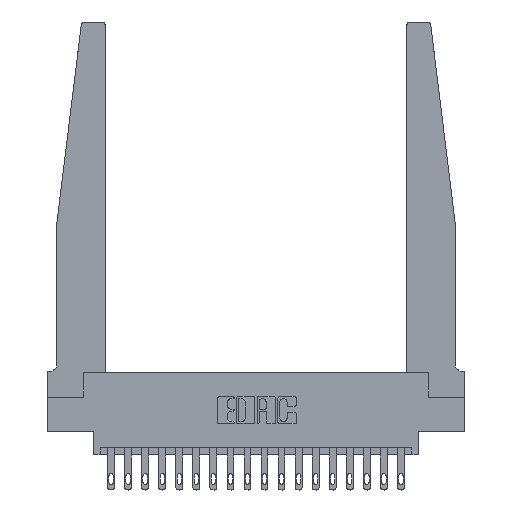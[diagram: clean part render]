
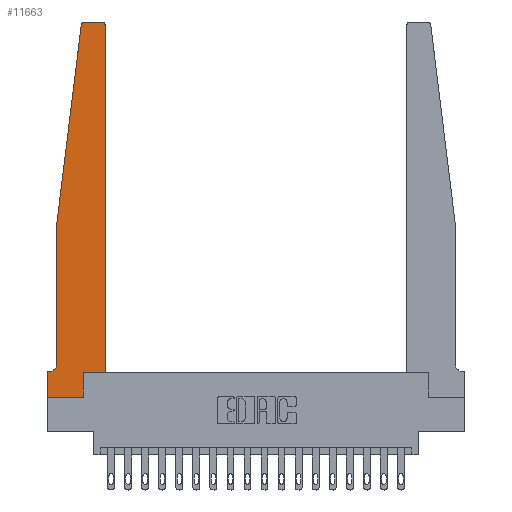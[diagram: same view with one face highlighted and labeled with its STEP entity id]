
A CAD part, top view. The second image highlights one B-rep face of the part: STEP entity #11663.
In plain terms, the highlighted planar face has unit normal (0, 0, 1).
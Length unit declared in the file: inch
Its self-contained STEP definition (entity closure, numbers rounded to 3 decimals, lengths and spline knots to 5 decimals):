
#493 = CARTESIAN_POINT ( 'NONE',  ( 0.425, 0.18, 0.37 ) ) ;
#527 = ORIENTED_EDGE ( 'NONE', *, *, #17623, .T. ) ;
#646 = LINE ( 'NONE', #11451, #14542 ) ;
#763 = LINE ( 'NONE', #2199, #16998 ) ;
#764 = LINE ( 'NONE', #10218, #9113 ) ;
#1046 = DIRECTION ( 'NONE',  ( 0., 0., 1. ) ) ;
#1295 = AXIS2_PLACEMENT_3D ( 'NONE', #3927, #1046, #13353 ) ;
#1672 = VECTOR ( 'NONE', #10915, 39.37008 ) ;
#1885 = EDGE_CURVE ( 'NONE', #11751, #8328, #15690, .T. ) ;
#2040 = LINE ( 'NONE', #493, #2294 ) ;
#2199 = CARTESIAN_POINT ( 'NONE',  ( 0.065, 1.25, 0.37 ) ) ;
#2294 = VECTOR ( 'NONE', #14551, 39.37008 ) ;
#2701 = EDGE_CURVE ( 'NONE', #14262, #3172, #12466, .T. ) ;
#2711 = ORIENTED_EDGE ( 'NONE', *, *, #9557, .T. ) ;
#2997 = PLANE ( 'NONE',  #3436 ) ;
#3044 = ORIENTED_EDGE ( 'NONE', *, *, #8744, .T. ) ;
#3060 = VECTOR ( 'NONE', #9280, 39.37008 ) ;
#3105 = LINE ( 'NONE', #9674, #11084 ) ;
#3172 = VERTEX_POINT ( 'NONE', #15794 ) ;
#3436 = AXIS2_PLACEMENT_3D ( 'NONE', #18452, #4448, #10693 ) ;
#3734 = VERTEX_POINT ( 'NONE', #14636 ) ;
#3927 = CARTESIAN_POINT ( 'NONE',  ( 0.395, 2.72, 0.37 ) ) ;
#4403 = EDGE_CURVE ( 'NONE', #17852, #5246, #763, .T. ) ;
#4408 = VERTEX_POINT ( 'NONE', #10315 ) ;
#4448 = DIRECTION ( 'NONE',  ( 0., 0., 1. ) ) ;
#4866 = CARTESIAN_POINT ( 'NONE',  ( 0., 0., 0.37 ) ) ;
#5148 = EDGE_CURVE ( 'NONE', #3734, #12328, #2040, .T. ) ;
#5246 = VERTEX_POINT ( 'NONE', #19945 ) ;
#5427 = AXIS2_PLACEMENT_3D ( 'NONE', #12506, #7591, #5840 ) ;
#5588 = AXIS2_PLACEMENT_3D ( 'NONE', #17784, #10431, #14735 ) ;
#5840 = DIRECTION ( 'NONE',  ( -1., 0., 0. ) ) ;
#5867 = EDGE_CURVE ( 'NONE', #3172, #17852, #6195, .T. ) ;
#6074 = VECTOR ( 'NONE', #16519, 39.37008 ) ;
#6195 = LINE ( 'NONE', #6605, #1672 ) ;
#6605 = CARTESIAN_POINT ( 'NONE',  ( 0.065, 1.25, 0.37 ) ) ;
#7305 = VERTEX_POINT ( 'NONE', #19201 ) ;
#7531 = FACE_OUTER_BOUND ( 'NONE', #16681, .T. ) ;
#7591 = DIRECTION ( 'NONE',  ( 0., 0., -1. ) ) ;
#7834 = DIRECTION ( 'NONE',  ( 1., 0., 0. ) ) ;
#8134 = ORIENTED_EDGE ( 'NONE', *, *, #10367, .T. ) ;
#8328 = VERTEX_POINT ( 'NONE', #20137 ) ;
#8391 = CARTESIAN_POINT ( 'NONE',  ( 0.2605, 0., 0.37 ) ) ;
#8435 = VECTOR ( 'NONE', #11987, 39.37008 ) ;
#8744 = EDGE_CURVE ( 'NONE', #7305, #4408, #14182, .T. ) ;
#9113 = VECTOR ( 'NONE', #11570, 39.37008 ) ;
#9280 = DIRECTION ( 'NONE',  ( 0., -1., 0. ) ) ;
#9557 = EDGE_CURVE ( 'NONE', #8328, #14262, #646, .T. ) ;
#9674 = CARTESIAN_POINT ( 'NONE',  ( 0., 0., 0.37 ) ) ;
#10131 = ORIENTED_EDGE ( 'NONE', *, *, #14165, .T. ) ;
#10218 = CARTESIAN_POINT ( 'NONE',  ( 0.2605, 0.18, 0.37 ) ) ;
#10315 = CARTESIAN_POINT ( 'NONE',  ( 0., 0., 0.37 ) ) ;
#10367 = EDGE_CURVE ( 'NONE', #18011, #7305, #17741, .T. ) ;
#10431 = DIRECTION ( 'NONE',  ( 0., 0., 1. ) ) ;
#10657 = CIRCLE ( 'NONE', #5427, 0.05 ) ;
#10693 = DIRECTION ( 'NONE',  ( 1., 0., 0. ) ) ;
#10798 = CARTESIAN_POINT ( 'NONE',  ( 0.425, 2.72, 0.37 ) ) ;
#10915 = DIRECTION ( 'NONE',  ( -0.122, -0.992, 0. ) ) ;
#11084 = VECTOR ( 'NONE', #7834, 39.37008 ) ;
#11189 = VERTEX_POINT ( 'NONE', #8391 ) ;
#11451 = CARTESIAN_POINT ( 'NONE',  ( 0.25, 2.75, 0.37 ) ) ;
#11553 = ORIENTED_EDGE ( 'NONE', *, *, #4403, .T. ) ;
#11570 = DIRECTION ( 'NONE',  ( 0., 1., 0. ) ) ;
#11663 = ADVANCED_FACE ( 'NONE', ( #7531 ), #2997, .T. ) ;
#11751 = VERTEX_POINT ( 'NONE', #10798 ) ;
#11837 = CARTESIAN_POINT ( 'NONE',  ( 0.065, 0.1875, 0.37 ) ) ;
#11987 = DIRECTION ( 'NONE',  ( 0., 1., 0. ) ) ;
#12049 = ORIENTED_EDGE ( 'NONE', *, *, #2701, .T. ) ;
#12328 = VERTEX_POINT ( 'NONE', #14745 ) ;
#12466 = CIRCLE ( 'NONE', #5588, 0.03 ) ;
#12506 = CARTESIAN_POINT ( 'NONE',  ( 0.015, 0.2375, 0.37 ) ) ;
#13353 = DIRECTION ( 'NONE',  ( 1., 0., 0. ) ) ;
#13857 = CARTESIAN_POINT ( 'NONE',  ( 0.065, 1.25, 0.37 ) ) ;
#13864 = ORIENTED_EDGE ( 'NONE', *, *, #5148, .T. ) ;
#14068 = ORIENTED_EDGE ( 'NONE', *, *, #17468, .T. ) ;
#14165 = EDGE_CURVE ( 'NONE', #5246, #18011, #10657, .T. ) ;
#14182 = LINE ( 'NONE', #4866, #3060 ) ;
#14262 = VERTEX_POINT ( 'NONE', #17476 ) ;
#14542 = VECTOR ( 'NONE', #19589, 39.37008 ) ;
#14551 = DIRECTION ( 'NONE',  ( 1., 0., 0. ) ) ;
#14585 = ORIENTED_EDGE ( 'NONE', *, *, #5867, .T. ) ;
#14636 = CARTESIAN_POINT ( 'NONE',  ( 0.2605, 0.18, 0.37 ) ) ;
#14735 = DIRECTION ( 'NONE',  ( 1., 0., 0. ) ) ;
#14745 = CARTESIAN_POINT ( 'NONE',  ( 0.425, 0.18, 0.37 ) ) ;
#15690 = CIRCLE ( 'NONE', #1295, 0.03 ) ;
#15794 = CARTESIAN_POINT ( 'NONE',  ( 0.24675, 2.72367, 0.37 ) ) ;
#16519 = DIRECTION ( 'NONE',  ( -1., 0., 0. ) ) ;
#16562 = LINE ( 'NONE', #19519, #8435 ) ;
#16681 = EDGE_LOOP ( 'NONE', ( #2711, #12049, #14585, #11553, #10131, #8134, #3044, #527, #14068, #13864, #18482, #18053 ) ) ;
#16998 = VECTOR ( 'NONE', #18075, 39.37008 ) ;
#17468 = EDGE_CURVE ( 'NONE', #11189, #3734, #764, .T. ) ;
#17476 = CARTESIAN_POINT ( 'NONE',  ( 0.27653, 2.75, 0.37 ) ) ;
#17623 = EDGE_CURVE ( 'NONE', #4408, #11189, #3105, .T. ) ;
#17716 = CARTESIAN_POINT ( 'NONE',  ( 0.015, 0.1875, 0.37 ) ) ;
#17741 = LINE ( 'NONE', #11837, #6074 ) ;
#17784 = CARTESIAN_POINT ( 'NONE',  ( 0.27653, 2.72, 0.37 ) ) ;
#17852 = VERTEX_POINT ( 'NONE', #13857 ) ;
#18011 = VERTEX_POINT ( 'NONE', #17716 ) ;
#18053 = ORIENTED_EDGE ( 'NONE', *, *, #1885, .T. ) ;
#18075 = DIRECTION ( 'NONE',  ( 0., -1., 0. ) ) ;
#18452 = CARTESIAN_POINT ( 'NONE',  ( 0., 0.1875, 0.37 ) ) ;
#18482 = ORIENTED_EDGE ( 'NONE', *, *, #18731, .T. ) ;
#18731 = EDGE_CURVE ( 'NONE', #12328, #11751, #16562, .T. ) ;
#19201 = CARTESIAN_POINT ( 'NONE',  ( 0., 0.1875, 0.37 ) ) ;
#19519 = CARTESIAN_POINT ( 'NONE',  ( 0.425, 0.18, 0.37 ) ) ;
#19589 = DIRECTION ( 'NONE',  ( -1., 0., 0. ) ) ;
#19945 = CARTESIAN_POINT ( 'NONE',  ( 0.065, 0.2375, 0.37 ) ) ;
#20137 = CARTESIAN_POINT ( 'NONE',  ( 0.395, 2.75, 0.37 ) ) ;
